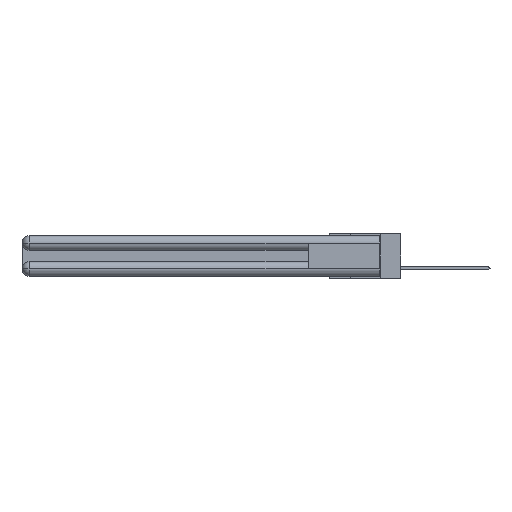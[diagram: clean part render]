
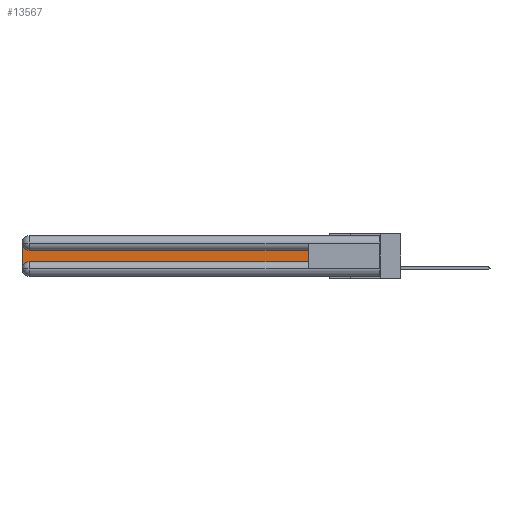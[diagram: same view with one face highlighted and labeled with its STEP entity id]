
A CAD part, left-side view. The second image highlights one B-rep face of the part: STEP entity #13567.
In plain terms, the highlighted planar face has unit normal (-1, 0, 0).
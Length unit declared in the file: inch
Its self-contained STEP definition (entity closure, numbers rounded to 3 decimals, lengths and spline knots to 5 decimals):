
#466 = PLANE ( 'NONE',  #11042 ) ;
#952 = VERTEX_POINT ( 'NONE', #29689 ) ;
#3159 = LINE ( 'NONE', #15080, #27149 ) ;
#3249 = EDGE_CURVE ( 'NONE', #7591, #17966, #12708, .T. ) ;
#3858 = ORIENTED_EDGE ( 'NONE', *, *, #31181, .T. ) ;
#4167 = CARTESIAN_POINT ( 'NONE',  ( 0.075, 2.94, -0.2775 ) ) ;
#4367 = CARTESIAN_POINT ( 'NONE',  ( 0.075, 0.6, -0.1225 ) ) ;
#4469 = CARTESIAN_POINT ( 'NONE',  ( 0.075, 2.94, -0.1225 ) ) ;
#4809 = CARTESIAN_POINT ( 'NONE',  ( 0.075, 2.94, -0.2175 ) ) ;
#7511 = VERTEX_POINT ( 'NONE', #21144 ) ;
#7591 = VERTEX_POINT ( 'NONE', #4809 ) ;
#8452 = DIRECTION ( 'NONE',  ( 0., -1., 0. ) ) ;
#8488 = EDGE_CURVE ( 'NONE', #17966, #952, #3159, .T. ) ;
#9550 = CIRCLE ( 'NONE', #12545, 0.06 ) ;
#10751 = DIRECTION ( 'NONE',  ( 0., 0., -1. ) ) ;
#10857 = CARTESIAN_POINT ( 'NONE',  ( 0.075, 2.94, -0.0625 ) ) ;
#10970 = DIRECTION ( 'NONE',  ( 1., 0., 0. ) ) ;
#11042 = AXIS2_PLACEMENT_3D ( 'NONE', #27319, #19690, #17529 ) ;
#11335 = ORIENTED_EDGE ( 'NONE', *, *, #12308, .T. ) ;
#12308 = EDGE_CURVE ( 'NONE', #952, #24438, #18189, .T. ) ;
#12545 = AXIS2_PLACEMENT_3D ( 'NONE', #4167, #26296, #26505 ) ;
#12708 = LINE ( 'NONE', #24802, #28735 ) ;
#13567 = ADVANCED_FACE ( 'NONE', ( #16644 ), #466, .F. ) ;
#13929 = ORIENTED_EDGE ( 'NONE', *, *, #14270, .T. ) ;
#14135 = AXIS2_PLACEMENT_3D ( 'NONE', #10857, #10970, #10751 ) ;
#14270 = EDGE_CURVE ( 'NONE', #7511, #24796, #16959, .T. ) ;
#14396 = ORIENTED_EDGE ( 'NONE', *, *, #16195, .T. ) ;
#14439 = CARTESIAN_POINT ( 'NONE',  ( 0.075, 3., -0.2175 ) ) ;
#15080 = CARTESIAN_POINT ( 'NONE',  ( 0.075, 0.6, -0.2175 ) ) ;
#16195 = EDGE_CURVE ( 'NONE', #24438, #7511, #22246, .T. ) ;
#16644 = FACE_OUTER_BOUND ( 'NONE', #27136, .T. ) ;
#16671 = ORIENTED_EDGE ( 'NONE', *, *, #8488, .T. ) ;
#16959 = LINE ( 'NONE', #14439, #31422 ) ;
#17172 = ORIENTED_EDGE ( 'NONE', *, *, #3249, .T. ) ;
#17529 = DIRECTION ( 'NONE',  ( 0., 0., -1. ) ) ;
#17966 = VERTEX_POINT ( 'NONE', #26069 ) ;
#17995 = DIRECTION ( 'NONE',  ( 0., 0., 1. ) ) ;
#18189 = LINE ( 'NONE', #4367, #26913 ) ;
#19690 = DIRECTION ( 'NONE',  ( 1., 0., 0. ) ) ;
#21144 = CARTESIAN_POINT ( 'NONE',  ( 0.075, 3., -0.0625 ) ) ;
#21418 = DIRECTION ( 'NONE',  ( 0., 1., 0. ) ) ;
#22246 = CIRCLE ( 'NONE', #14135, 0.06 ) ;
#23864 = DIRECTION ( 'NONE',  ( 0., 0., -1. ) ) ;
#24438 = VERTEX_POINT ( 'NONE', #4469 ) ;
#24796 = VERTEX_POINT ( 'NONE', #30478 ) ;
#24802 = CARTESIAN_POINT ( 'NONE',  ( 0.075, 0.6, -0.2175 ) ) ;
#26069 = CARTESIAN_POINT ( 'NONE',  ( 0.075, 0.6, -0.2175 ) ) ;
#26296 = DIRECTION ( 'NONE',  ( 1., 0., 0. ) ) ;
#26505 = DIRECTION ( 'NONE',  ( 0., 0., -1. ) ) ;
#26913 = VECTOR ( 'NONE', #21418, 39.37008 ) ;
#27136 = EDGE_LOOP ( 'NONE', ( #11335, #14396, #13929, #3858, #17172, #16671 ) ) ;
#27149 = VECTOR ( 'NONE', #17995, 39.37008 ) ;
#27319 = CARTESIAN_POINT ( 'NONE',  ( 0.075, 3., -0.1225 ) ) ;
#28735 = VECTOR ( 'NONE', #8452, 39.37008 ) ;
#29689 = CARTESIAN_POINT ( 'NONE',  ( 0.075, 0.6, -0.1225 ) ) ;
#30478 = CARTESIAN_POINT ( 'NONE',  ( 0.075, 3., -0.2775 ) ) ;
#31181 = EDGE_CURVE ( 'NONE', #24796, #7591, #9550, .T. ) ;
#31422 = VECTOR ( 'NONE', #23864, 39.37008 ) ;
